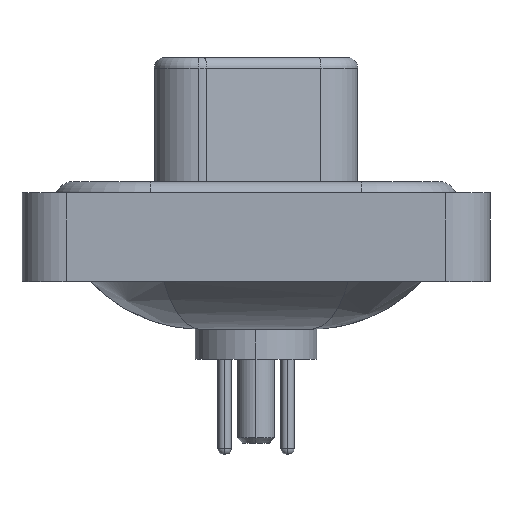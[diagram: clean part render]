
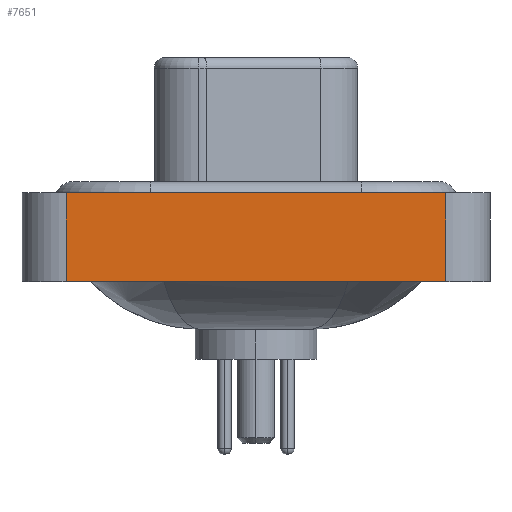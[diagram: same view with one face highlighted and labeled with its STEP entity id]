
A CAD part, left-side view. The second image highlights one B-rep face of the part: STEP entity #7651.
In plain terms, the highlighted planar face has unit normal (-1, 0, 0).
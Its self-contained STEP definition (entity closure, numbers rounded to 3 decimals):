
#30 = ORIENTED_EDGE ( 'NONE', *, *, #6127, .F. ) ;
#786 = ORIENTED_EDGE ( 'NONE', *, *, #10453, .T. ) ;
#901 = VECTOR ( 'NONE', #16917, 1000. ) ;
#2144 = VECTOR ( 'NONE', #14602, 1000. ) ;
#3335 = EDGE_LOOP ( 'NONE', ( #10668, #30, #7371, #786 ) ) ;
#3725 = CARTESIAN_POINT ( 'NONE',  ( -7.3, 8.55, -3.6 ) ) ;
#4162 = CARTESIAN_POINT ( 'NONE',  ( -7.3, -8.55, -3.6 ) ) ;
#4214 = CARTESIAN_POINT ( 'NONE',  ( -7.3, -8.55, 0.4 ) ) ;
#4491 = CARTESIAN_POINT ( 'NONE',  ( -7.3, -8.55, 0.4 ) ) ;
#5555 = LINE ( 'NONE', #4214, #2144 ) ;
#5952 = EDGE_CURVE ( 'NONE', #14490, #15743, #16635, .T. ) ;
#6127 = EDGE_CURVE ( 'NONE', #15743, #17694, #5555, .T. ) ;
#7371 = ORIENTED_EDGE ( 'NONE', *, *, #5952, .F. ) ;
#7651 = ADVANCED_FACE ( 'NONE', ( #14451 ), #16187, .T. ) ;
#8065 = AXIS2_PLACEMENT_3D ( 'NONE', #11818, #17625, #17730 ) ;
#8649 = DIRECTION ( 'NONE',  ( 0., 0., 1. ) ) ;
#9898 = CARTESIAN_POINT ( 'NONE',  ( -7.3, 8.55, 0.4 ) ) ;
#10453 = EDGE_CURVE ( 'NONE', #14490, #18825, #10537, .T. ) ;
#10537 = LINE ( 'NONE', #4162, #17557 ) ;
#10668 = ORIENTED_EDGE ( 'NONE', *, *, #14263, .T. ) ;
#10725 = VECTOR ( 'NONE', #8649, 1000. ) ;
#11818 = CARTESIAN_POINT ( 'NONE',  ( -7.3, -8.55, -3.6 ) ) ;
#11996 = DIRECTION ( 'NONE',  ( 0., -1., 0. ) ) ;
#12871 = CARTESIAN_POINT ( 'NONE',  ( -7.3, 8.55, -3.6 ) ) ;
#13148 = CARTESIAN_POINT ( 'NONE',  ( -7.3, -8.55, -3.6 ) ) ;
#14263 = EDGE_CURVE ( 'NONE', #18825, #17694, #17384, .T. ) ;
#14451 = FACE_OUTER_BOUND ( 'NONE', #3335, .T. ) ;
#14490 = VERTEX_POINT ( 'NONE', #12871 ) ;
#14602 = DIRECTION ( 'NONE',  ( 0., -1., 0. ) ) ;
#15743 = VERTEX_POINT ( 'NONE', #9898 ) ;
#16187 = PLANE ( 'NONE',  #8065 ) ;
#16635 = LINE ( 'NONE', #3725, #901 ) ;
#16917 = DIRECTION ( 'NONE',  ( 0., 0., 1. ) ) ;
#17384 = LINE ( 'NONE', #13148, #10725 ) ;
#17557 = VECTOR ( 'NONE', #11996, 1000. ) ;
#17625 = DIRECTION ( 'NONE',  ( -1., 0., 0. ) ) ;
#17694 = VERTEX_POINT ( 'NONE', #4491 ) ;
#17730 = DIRECTION ( 'NONE',  ( 0., 0., 1. ) ) ;
#18825 = VERTEX_POINT ( 'NONE', #18973 ) ;
#18973 = CARTESIAN_POINT ( 'NONE',  ( -7.3, -8.55, -3.6 ) ) ;
